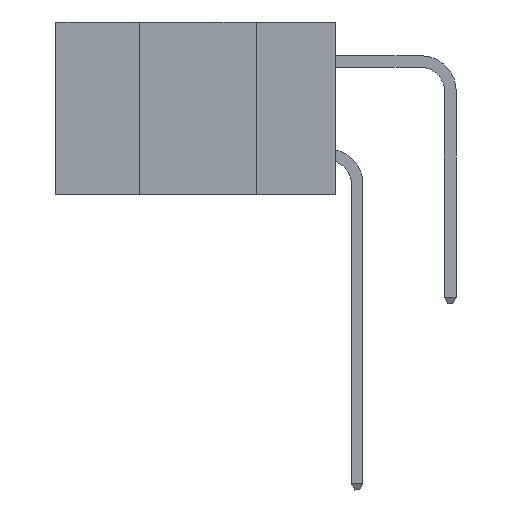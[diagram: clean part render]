
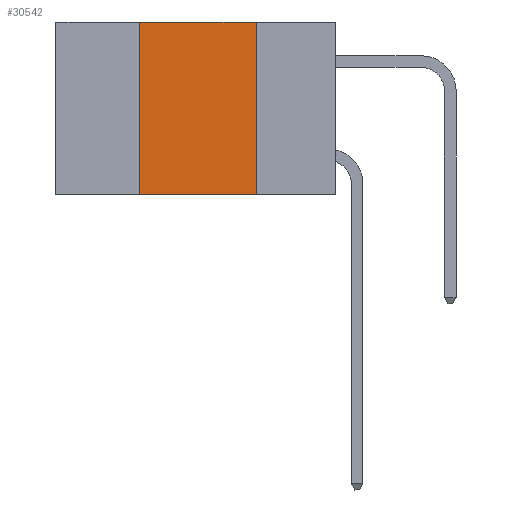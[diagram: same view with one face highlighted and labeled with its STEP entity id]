
A CAD part, left-side view. The second image highlights one B-rep face of the part: STEP entity #30542.
In plain terms, the highlighted planar face has unit normal (-1, 0, 0).
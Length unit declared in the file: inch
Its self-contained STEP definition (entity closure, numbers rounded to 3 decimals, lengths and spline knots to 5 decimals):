
#232 = FACE_OUTER_BOUND ( 'NONE', #13825, .T. ) ;
#415 = CARTESIAN_POINT ( 'NONE',  ( 0., 0.6, 0. ) ) ;
#924 = EDGE_CURVE ( 'NONE', #15794, #20202, #15200, .T. ) ;
#2763 = CARTESIAN_POINT ( 'NONE',  ( 0., 0.42, 0. ) ) ;
#2894 = ORIENTED_EDGE ( 'NONE', *, *, #15404, .F. ) ;
#3248 = EDGE_CURVE ( 'NONE', #33583, #20202, #31799, .T. ) ;
#4620 = ORIENTED_EDGE ( 'NONE', *, *, #29420, .F. ) ;
#4923 = VECTOR ( 'NONE', #19215, 39.37008 ) ;
#6464 = ORIENTED_EDGE ( 'NONE', *, *, #924, .T. ) ;
#7666 = DIRECTION ( 'NONE',  ( 0., -1., 0. ) ) ;
#8825 = CARTESIAN_POINT ( 'NONE',  ( 0., 0.17, -0.37 ) ) ;
#9790 = CARTESIAN_POINT ( 'NONE',  ( 0., 0.17, 0. ) ) ;
#11333 = VECTOR ( 'NONE', #26803, 39.37008 ) ;
#12498 = LINE ( 'NONE', #415, #4923 ) ;
#13211 = CARTESIAN_POINT ( 'NONE',  ( 0., 0.6, -0.37 ) ) ;
#13825 = EDGE_LOOP ( 'NONE', ( #14517, #2894, #4620, #6464 ) ) ;
#14250 = CARTESIAN_POINT ( 'NONE',  ( 0., 0.42, 0. ) ) ;
#14517 = ORIENTED_EDGE ( 'NONE', *, *, #3248, .F. ) ;
#15200 = LINE ( 'NONE', #13211, #19341 ) ;
#15404 = EDGE_CURVE ( 'NONE', #21665, #33583, #12498, .T. ) ;
#15794 = VERTEX_POINT ( 'NONE', #22938 ) ;
#17700 = DIRECTION ( 'NONE',  ( 0., 0., -1. ) ) ;
#19215 = DIRECTION ( 'NONE',  ( 0., -1., 0. ) ) ;
#19341 = VECTOR ( 'NONE', #7666, 39.37008 ) ;
#20050 = VECTOR ( 'NONE', #30472, 39.37008 ) ;
#20202 = VERTEX_POINT ( 'NONE', #8825 ) ;
#21665 = VERTEX_POINT ( 'NONE', #14250 ) ;
#22938 = CARTESIAN_POINT ( 'NONE',  ( 0., 0.42, -0.37 ) ) ;
#23070 = PLANE ( 'NONE',  #32299 ) ;
#23309 = DIRECTION ( 'NONE',  ( 1., 0., 0. ) ) ;
#23530 = LINE ( 'NONE', #2763, #11333 ) ;
#26803 = DIRECTION ( 'NONE',  ( 0., 0., 1. ) ) ;
#29420 = EDGE_CURVE ( 'NONE', #15794, #21665, #23530, .T. ) ;
#30472 = DIRECTION ( 'NONE',  ( 0., 0., -1. ) ) ;
#30542 = ADVANCED_FACE ( 'NONE', ( #232 ), #23070, .F. ) ;
#31799 = LINE ( 'NONE', #32931, #20050 ) ;
#32299 = AXIS2_PLACEMENT_3D ( 'NONE', #34090, #23309, #17700 ) ;
#32931 = CARTESIAN_POINT ( 'NONE',  ( 0., 0.17, 0. ) ) ;
#33583 = VERTEX_POINT ( 'NONE', #9790 ) ;
#34090 = CARTESIAN_POINT ( 'NONE',  ( 0., 0.6, 0. ) ) ;
